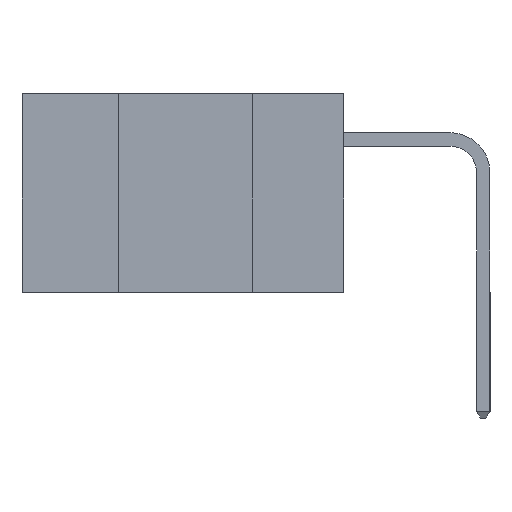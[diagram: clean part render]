
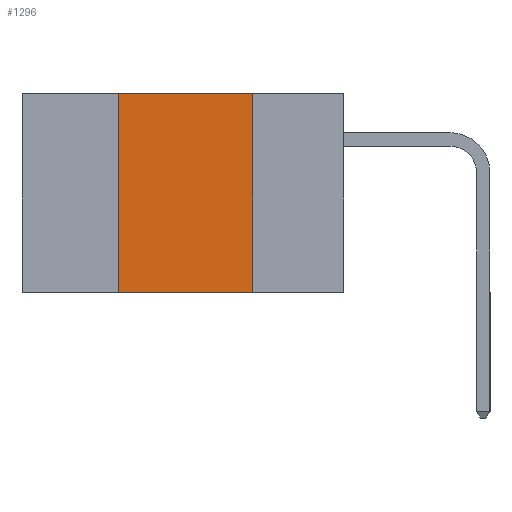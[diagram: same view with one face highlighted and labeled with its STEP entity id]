
A CAD part, left-side view. The second image highlights one B-rep face of the part: STEP entity #1296.
In plain terms, the highlighted planar face has unit normal (-1, 0, 0).
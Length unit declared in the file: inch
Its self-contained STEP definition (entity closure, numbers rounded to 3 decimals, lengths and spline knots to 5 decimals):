
#780 = CARTESIAN_POINT ( 'NONE',  ( 0., 0.42, -0.37 ) ) ;
#1296 = ADVANCED_FACE ( 'NONE', ( #4063 ), #2254, .F. ) ;
#2074 = CARTESIAN_POINT ( 'NONE',  ( 0., 0.42, 0. ) ) ;
#2254 = PLANE ( 'NONE',  #9690 ) ;
#2445 = ORIENTED_EDGE ( 'NONE', *, *, #15061, .F. ) ;
#2678 = VECTOR ( 'NONE', #14989, 39.37008 ) ;
#2924 = DIRECTION ( 'NONE',  ( 0., -1., 0. ) ) ;
#3401 = ORIENTED_EDGE ( 'NONE', *, *, #10576, .F. ) ;
#3597 = DIRECTION ( 'NONE',  ( 0., 0., 1. ) ) ;
#3823 = CARTESIAN_POINT ( 'NONE',  ( 0., 0.42, 0. ) ) ;
#4063 = FACE_OUTER_BOUND ( 'NONE', #16608, .T. ) ;
#4596 = VERTEX_POINT ( 'NONE', #17891 ) ;
#4648 = LINE ( 'NONE', #17209, #16342 ) ;
#4797 = DIRECTION ( 'NONE',  ( 1., 0., 0. ) ) ;
#6239 = CARTESIAN_POINT ( 'NONE',  ( 0., 0.17, 0. ) ) ;
#6272 = ORIENTED_EDGE ( 'NONE', *, *, #11210, .T. ) ;
#6836 = LINE ( 'NONE', #2074, #17962 ) ;
#8071 = CARTESIAN_POINT ( 'NONE',  ( 0., 0.6, 0. ) ) ;
#8511 = DIRECTION ( 'NONE',  ( 0., -1., 0. ) ) ;
#9690 = AXIS2_PLACEMENT_3D ( 'NONE', #8071, #4797, #17216 ) ;
#10576 = EDGE_CURVE ( 'NONE', #16360, #13926, #4648, .T. ) ;
#10663 = LINE ( 'NONE', #6239, #2678 ) ;
#11210 = EDGE_CURVE ( 'NONE', #15328, #4596, #16083, .T. ) ;
#12253 = VECTOR ( 'NONE', #2924, 39.37008 ) ;
#12255 = ORIENTED_EDGE ( 'NONE', *, *, #18735, .F. ) ;
#13926 = VERTEX_POINT ( 'NONE', #17915 ) ;
#14989 = DIRECTION ( 'NONE',  ( 0., 0., -1. ) ) ;
#15061 = EDGE_CURVE ( 'NONE', #13926, #4596, #10663, .T. ) ;
#15328 = VERTEX_POINT ( 'NONE', #780 ) ;
#16083 = LINE ( 'NONE', #19046, #12253 ) ;
#16342 = VECTOR ( 'NONE', #8511, 39.37008 ) ;
#16360 = VERTEX_POINT ( 'NONE', #3823 ) ;
#16608 = EDGE_LOOP ( 'NONE', ( #2445, #3401, #12255, #6272 ) ) ;
#17209 = CARTESIAN_POINT ( 'NONE',  ( 0., 0.6, 0. ) ) ;
#17216 = DIRECTION ( 'NONE',  ( 0., 0., -1. ) ) ;
#17891 = CARTESIAN_POINT ( 'NONE',  ( 0., 0.17, -0.37 ) ) ;
#17915 = CARTESIAN_POINT ( 'NONE',  ( 0., 0.17, 0. ) ) ;
#17962 = VECTOR ( 'NONE', #3597, 39.37008 ) ;
#18735 = EDGE_CURVE ( 'NONE', #15328, #16360, #6836, .T. ) ;
#19046 = CARTESIAN_POINT ( 'NONE',  ( 0., 0.6, -0.37 ) ) ;
